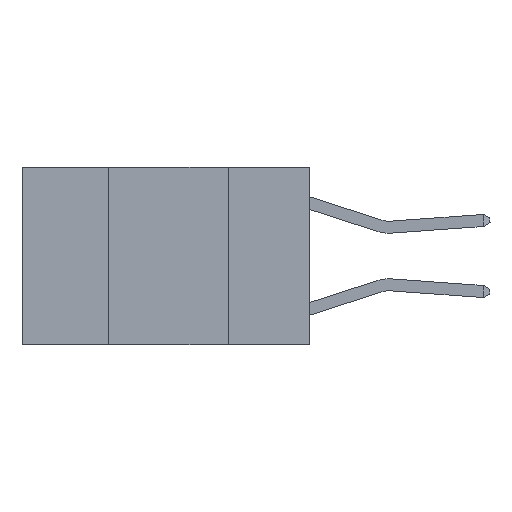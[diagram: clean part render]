
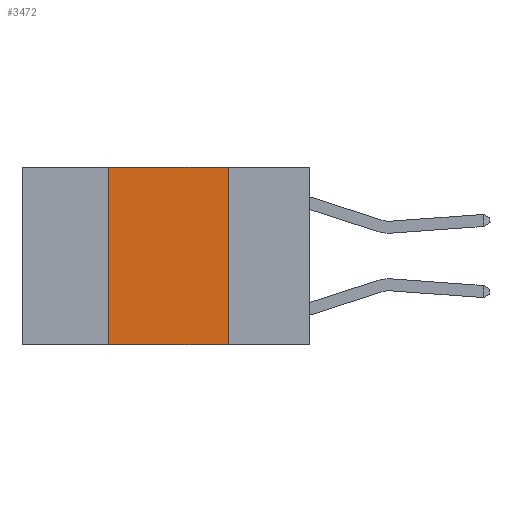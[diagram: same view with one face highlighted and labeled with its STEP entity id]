
A CAD part, left-side view. The second image highlights one B-rep face of the part: STEP entity #3472.
In plain terms, the highlighted planar face has unit normal (-1, 0, 0).
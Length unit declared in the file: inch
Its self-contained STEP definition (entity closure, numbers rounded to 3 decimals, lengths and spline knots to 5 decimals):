
#145 = EDGE_CURVE ( 'NONE', #7016, #2369, #2305, .T. ) ;
#426 = DIRECTION ( 'NONE',  ( 0., -1., 0. ) ) ;
#722 = FACE_OUTER_BOUND ( 'NONE', #2658, .T. ) ;
#1239 = EDGE_CURVE ( 'NONE', #2369, #8498, #3811, .T. ) ;
#1314 = CARTESIAN_POINT ( 'NONE',  ( 0., 0.17, -0.37 ) ) ;
#2145 = AXIS2_PLACEMENT_3D ( 'NONE', #2560, #2549, #2531 ) ;
#2305 = LINE ( 'NONE', #9165, #2388 ) ;
#2347 = VECTOR ( 'NONE', #426, 39.37008 ) ;
#2369 = VERTEX_POINT ( 'NONE', #6534 ) ;
#2388 = VECTOR ( 'NONE', #9182, 39.37008 ) ;
#2531 = DIRECTION ( 'NONE',  ( 0., 0., -1. ) ) ;
#2549 = DIRECTION ( 'NONE',  ( 1., 0., 0. ) ) ;
#2560 = CARTESIAN_POINT ( 'NONE',  ( 0., 0.6, 0. ) ) ;
#2609 = LINE ( 'NONE', #3795, #2347 ) ;
#2644 = PLANE ( 'NONE',  #2145 ) ;
#2658 = EDGE_LOOP ( 'NONE', ( #4011, #4032, #4055, #4102 ) ) ;
#3268 = CARTESIAN_POINT ( 'NONE',  ( 0., 0.42, -0.37 ) ) ;
#3472 = ADVANCED_FACE ( 'NONE', ( #722 ), #2644, .F. ) ;
#3795 = CARTESIAN_POINT ( 'NONE',  ( 0., 0.6, -0.37 ) ) ;
#3811 = LINE ( 'NONE', #7773, #5422 ) ;
#4011 = ORIENTED_EDGE ( 'NONE', *, *, #1239, .F. ) ;
#4032 = ORIENTED_EDGE ( 'NONE', *, *, #145, .F. ) ;
#4055 = ORIENTED_EDGE ( 'NONE', *, *, #8347, .F. ) ;
#4102 = ORIENTED_EDGE ( 'NONE', *, *, #8349, .T. ) ;
#4568 = CARTESIAN_POINT ( 'NONE',  ( 0., 0.42, 0. ) ) ;
#5386 = DIRECTION ( 'NONE',  ( 0., 0., 1. ) ) ;
#5422 = VECTOR ( 'NONE', #5699, 39.37008 ) ;
#5544 = VERTEX_POINT ( 'NONE', #3268 ) ;
#5699 = DIRECTION ( 'NONE',  ( 0., 0., -1. ) ) ;
#5877 = CARTESIAN_POINT ( 'NONE',  ( 0., 0.42, 0. ) ) ;
#6534 = CARTESIAN_POINT ( 'NONE',  ( 0., 0.17, 0. ) ) ;
#6635 = VECTOR ( 'NONE', #5386, 39.37008 ) ;
#6874 = LINE ( 'NONE', #4568, #6635 ) ;
#7016 = VERTEX_POINT ( 'NONE', #5877 ) ;
#7773 = CARTESIAN_POINT ( 'NONE',  ( 0., 0.17, 0. ) ) ;
#8347 = EDGE_CURVE ( 'NONE', #5544, #7016, #6874, .T. ) ;
#8349 = EDGE_CURVE ( 'NONE', #5544, #8498, #2609, .T. ) ;
#8498 = VERTEX_POINT ( 'NONE', #1314 ) ;
#9165 = CARTESIAN_POINT ( 'NONE',  ( 0., 0.6, 0. ) ) ;
#9182 = DIRECTION ( 'NONE',  ( 0., -1., 0. ) ) ;
